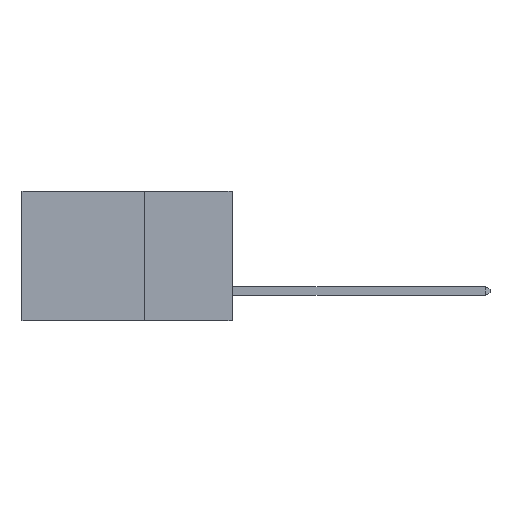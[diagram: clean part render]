
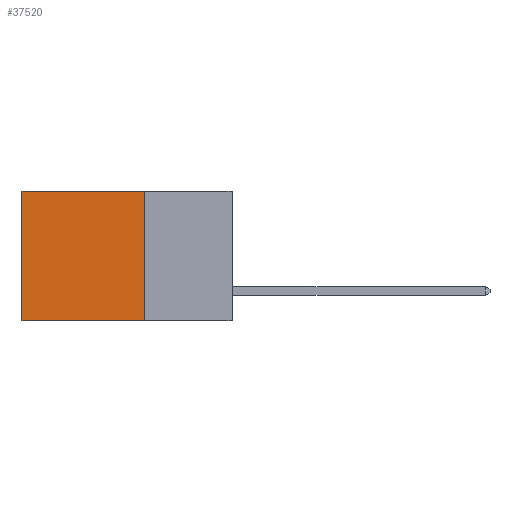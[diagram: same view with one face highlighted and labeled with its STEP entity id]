
A CAD part, left-side view. The second image highlights one B-rep face of the part: STEP entity #37520.
In plain terms, the highlighted planar face has unit normal (-1, 0, 0).
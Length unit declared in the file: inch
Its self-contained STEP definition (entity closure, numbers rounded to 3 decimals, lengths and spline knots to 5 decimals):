
#1078 = LINE ( 'NONE', #28252, #32247 ) ;
#2425 = DIRECTION ( 'NONE',  ( 0., 0., -1. ) ) ;
#3793 = CARTESIAN_POINT ( 'NONE',  ( 0.2875, 0.6, 0. ) ) ;
#5505 = EDGE_CURVE ( 'NONE', #25097, #16094, #1078, .T. ) ;
#5945 = DIRECTION ( 'NONE',  ( 1., 0., 0. ) ) ;
#6019 = EDGE_CURVE ( 'NONE', #32592, #35765, #14283, .T. ) ;
#6455 = DIRECTION ( 'NONE',  ( 0., 1., 0. ) ) ;
#7148 = AXIS2_PLACEMENT_3D ( 'NONE', #24193, #5945, #27195 ) ;
#10467 = VECTOR ( 'NONE', #2425, 39.37008 ) ;
#11230 = CARTESIAN_POINT ( 'NONE',  ( 0.2875, 0.25, -0.37 ) ) ;
#12030 = ORIENTED_EDGE ( 'NONE', *, *, #16807, .F. ) ;
#14283 = LINE ( 'NONE', #18638, #37331 ) ;
#15007 = PLANE ( 'NONE',  #7148 ) ;
#16094 = VERTEX_POINT ( 'NONE', #20538 ) ;
#16807 = EDGE_CURVE ( 'NONE', #32592, #25097, #25700, .T. ) ;
#17122 = CARTESIAN_POINT ( 'NONE',  ( 0.2875, 0.6, 0. ) ) ;
#18638 = CARTESIAN_POINT ( 'NONE',  ( 0.2875, 0.25, 0. ) ) ;
#19201 = VECTOR ( 'NONE', #31012, 39.37008 ) ;
#20538 = CARTESIAN_POINT ( 'NONE',  ( 0.2875, 0.6, -0.37 ) ) ;
#21509 = CARTESIAN_POINT ( 'NONE',  ( 0.2875, 0.25, 0. ) ) ;
#22193 = EDGE_CURVE ( 'NONE', #35765, #16094, #27166, .T. ) ;
#23699 = ORIENTED_EDGE ( 'NONE', *, *, #5505, .F. ) ;
#24193 = CARTESIAN_POINT ( 'NONE',  ( 0.2875, 0.25, 0. ) ) ;
#25097 = VERTEX_POINT ( 'NONE', #11230 ) ;
#25700 = LINE ( 'NONE', #29508, #10467 ) ;
#27166 = LINE ( 'NONE', #3793, #19201 ) ;
#27195 = DIRECTION ( 'NONE',  ( 0., 0., -1. ) ) ;
#27750 = EDGE_LOOP ( 'NONE', ( #38786, #23699, #12030, #34477 ) ) ;
#28252 = CARTESIAN_POINT ( 'NONE',  ( 0.2875, 0.25, -0.37 ) ) ;
#29508 = CARTESIAN_POINT ( 'NONE',  ( 0.2875, 0.25, 0. ) ) ;
#31012 = DIRECTION ( 'NONE',  ( 0., 0., -1. ) ) ;
#31239 = DIRECTION ( 'NONE',  ( 0., 1., 0. ) ) ;
#32247 = VECTOR ( 'NONE', #31239, 39.37008 ) ;
#32592 = VERTEX_POINT ( 'NONE', #21509 ) ;
#34477 = ORIENTED_EDGE ( 'NONE', *, *, #6019, .T. ) ;
#34770 = FACE_OUTER_BOUND ( 'NONE', #27750, .T. ) ;
#35765 = VERTEX_POINT ( 'NONE', #17122 ) ;
#37331 = VECTOR ( 'NONE', #6455, 39.37008 ) ;
#37520 = ADVANCED_FACE ( 'NONE', ( #34770 ), #15007, .F. ) ;
#38786 = ORIENTED_EDGE ( 'NONE', *, *, #22193, .T. ) ;
